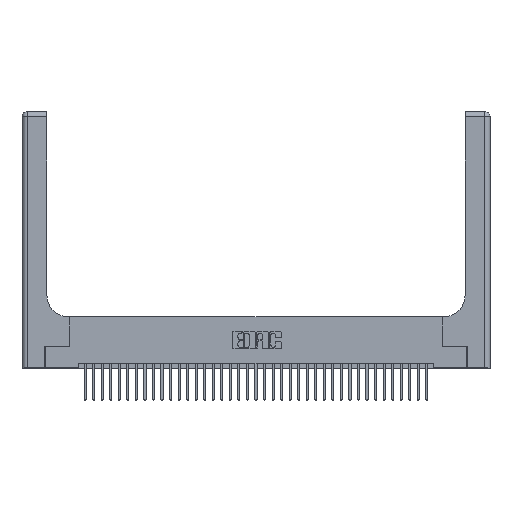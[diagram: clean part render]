
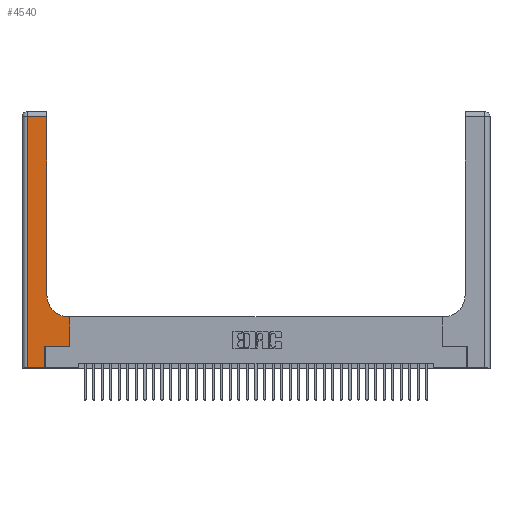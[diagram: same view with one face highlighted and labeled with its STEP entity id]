
A CAD part, top view. The second image highlights one B-rep face of the part: STEP entity #4540.
In plain terms, the highlighted planar face has unit normal (0, 0, 1).
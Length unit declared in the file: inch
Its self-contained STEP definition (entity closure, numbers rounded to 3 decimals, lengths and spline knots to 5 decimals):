
#479 = CARTESIAN_POINT ( 'NONE',  ( 0.5585, 0.25, 0.37 ) ) ;
#609 = CARTESIAN_POINT ( 'NONE',  ( 0.2915, 2.94, 0.37 ) ) ;
#847 = ORIENTED_EDGE ( 'NONE', *, *, #27261, .T. ) ;
#1222 = VERTEX_POINT ( 'NONE', #27200 ) ;
#1748 = DIRECTION ( 'NONE',  ( -1., 0., 0. ) ) ;
#1931 = VERTEX_POINT ( 'NONE', #24412 ) ;
#3853 = VECTOR ( 'NONE', #25862, 39.37008 ) ;
#4018 = VERTEX_POINT ( 'NONE', #5456 ) ;
#4540 = ADVANCED_FACE ( 'NONE', ( #33592 ), #36421, .F. ) ;
#4553 = CARTESIAN_POINT ( 'NONE',  ( 0., 0., 0.37 ) ) ;
#5456 = CARTESIAN_POINT ( 'NONE',  ( 0.06, 0., 0.37 ) ) ;
#5984 = ORIENTED_EDGE ( 'NONE', *, *, #18983, .T. ) ;
#6249 = LINE ( 'NONE', #479, #36906 ) ;
#7385 = EDGE_CURVE ( 'NONE', #13070, #31162, #11771, .T. ) ;
#8035 = DIRECTION ( 'NONE',  ( 0., -1., 0. ) ) ;
#8072 = VERTEX_POINT ( 'NONE', #32375 ) ;
#9146 = CARTESIAN_POINT ( 'NONE',  ( 0.5415, 0.85, 0.37 ) ) ;
#10310 = EDGE_CURVE ( 'NONE', #13200, #8072, #11595, .T. ) ;
#10456 = VECTOR ( 'NONE', #17176, 39.37008 ) ;
#11319 = EDGE_CURVE ( 'NONE', #4018, #1931, #32600, .T. ) ;
#11595 = CIRCLE ( 'NONE', #12958, 0.25 ) ;
#11771 = LINE ( 'NONE', #23020, #3853 ) ;
#11866 = ORIENTED_EDGE ( 'NONE', *, *, #22556, .T. ) ;
#12152 = DIRECTION ( 'NONE',  ( 1., 0., 0. ) ) ;
#12958 = AXIS2_PLACEMENT_3D ( 'NONE', #9146, #29326, #12152 ) ;
#13070 = VERTEX_POINT ( 'NONE', #609 ) ;
#13200 = VERTEX_POINT ( 'NONE', #25065 ) ;
#13995 = DIRECTION ( 'NONE',  ( 0., 1., 0. ) ) ;
#14261 = CARTESIAN_POINT ( 'NONE',  ( 0.269, 0.25, 0.37 ) ) ;
#14758 = VECTOR ( 'NONE', #19780, 39.37008 ) ;
#16646 = CARTESIAN_POINT ( 'NONE',  ( 0.2915, 3., 0.37 ) ) ;
#17176 = DIRECTION ( 'NONE',  ( 1., 0., 0. ) ) ;
#18783 = VECTOR ( 'NONE', #13995, 39.37008 ) ;
#18983 = EDGE_CURVE ( 'NONE', #1222, #26147, #6249, .T. ) ;
#19414 = DIRECTION ( 'NONE',  ( 0., 0., -1. ) ) ;
#19529 = DIRECTION ( 'NONE',  ( 0., 1., 0. ) ) ;
#19780 = DIRECTION ( 'NONE',  ( -1., 0., 0. ) ) ;
#19933 = EDGE_CURVE ( 'NONE', #8072, #13070, #35937, .T. ) ;
#19950 = ORIENTED_EDGE ( 'NONE', *, *, #10310, .T. ) ;
#20494 = ORIENTED_EDGE ( 'NONE', *, *, #11319, .T. ) ;
#20765 = CARTESIAN_POINT ( 'NONE',  ( 0.269, 0.25, 0.37 ) ) ;
#21099 = DIRECTION ( 'NONE',  ( 0., 1., 0. ) ) ;
#21988 = DIRECTION ( 'NONE',  ( 1., 0., 0. ) ) ;
#22440 = LINE ( 'NONE', #33909, #14758 ) ;
#22556 = EDGE_CURVE ( 'NONE', #26147, #13200, #22440, .T. ) ;
#23020 = CARTESIAN_POINT ( 'NONE',  ( 0., 2.94, 0.37 ) ) ;
#23238 = CARTESIAN_POINT ( 'NONE',  ( 0.06, 2.94, 0.37 ) ) ;
#23415 = ORIENTED_EDGE ( 'NONE', *, *, #19933, .T. ) ;
#23545 = ORIENTED_EDGE ( 'NONE', *, *, #24998, .T. ) ;
#24412 = CARTESIAN_POINT ( 'NONE',  ( 0.269, 0., 0.37 ) ) ;
#24998 = EDGE_CURVE ( 'NONE', #31162, #4018, #36476, .T. ) ;
#25065 = CARTESIAN_POINT ( 'NONE',  ( 0.5415, 0.6, 0.37 ) ) ;
#25441 = CARTESIAN_POINT ( 'NONE',  ( 0.06, 3., 0.37 ) ) ;
#25862 = DIRECTION ( 'NONE',  ( -1., 0., 0. ) ) ;
#26058 = VERTEX_POINT ( 'NONE', #20765 ) ;
#26147 = VERTEX_POINT ( 'NONE', #32542 ) ;
#26349 = AXIS2_PLACEMENT_3D ( 'NONE', #33564, #19414, #1748 ) ;
#26372 = LINE ( 'NONE', #36810, #18783 ) ;
#27200 = CARTESIAN_POINT ( 'NONE',  ( 0.5585, 0.25, 0.37 ) ) ;
#27261 = EDGE_CURVE ( 'NONE', #26058, #1222, #27618, .T. ) ;
#27618 = LINE ( 'NONE', #14261, #10456 ) ;
#29326 = DIRECTION ( 'NONE',  ( 0., 0., -1. ) ) ;
#30110 = ORIENTED_EDGE ( 'NONE', *, *, #7385, .T. ) ;
#31162 = VERTEX_POINT ( 'NONE', #23238 ) ;
#31732 = VECTOR ( 'NONE', #21988, 39.37008 ) ;
#32375 = CARTESIAN_POINT ( 'NONE',  ( 0.2915, 0.85, 0.37 ) ) ;
#32517 = EDGE_CURVE ( 'NONE', #1931, #26058, #26372, .T. ) ;
#32542 = CARTESIAN_POINT ( 'NONE',  ( 0.5585, 0.6, 0.37 ) ) ;
#32600 = LINE ( 'NONE', #4553, #31732 ) ;
#33564 = CARTESIAN_POINT ( 'NONE',  ( 0., 3., 0.37 ) ) ;
#33592 = FACE_OUTER_BOUND ( 'NONE', #34884, .T. ) ;
#33909 = CARTESIAN_POINT ( 'NONE',  ( 0.2915, 0.6, 0.37 ) ) ;
#34771 = ORIENTED_EDGE ( 'NONE', *, *, #32517, .T. ) ;
#34884 = EDGE_LOOP ( 'NONE', ( #23415, #30110, #23545, #20494, #34771, #847, #5984, #11866, #19950 ) ) ;
#35049 = VECTOR ( 'NONE', #19529, 39.37008 ) ;
#35937 = LINE ( 'NONE', #16646, #35049 ) ;
#36421 = PLANE ( 'NONE',  #26349 ) ;
#36476 = LINE ( 'NONE', #25441, #37354 ) ;
#36810 = CARTESIAN_POINT ( 'NONE',  ( 0.269, 0., 0.37 ) ) ;
#36906 = VECTOR ( 'NONE', #21099, 39.37008 ) ;
#37354 = VECTOR ( 'NONE', #8035, 39.37008 ) ;
